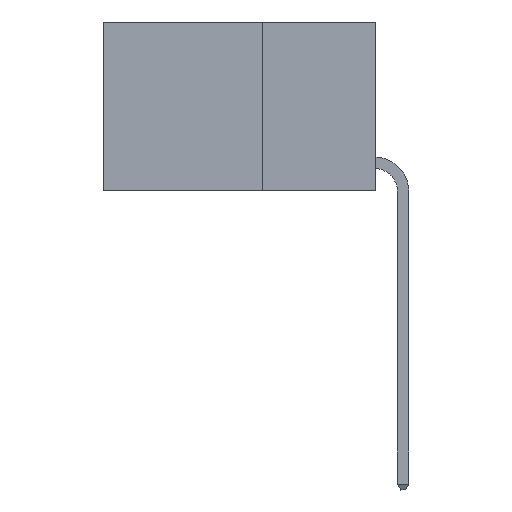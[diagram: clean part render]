
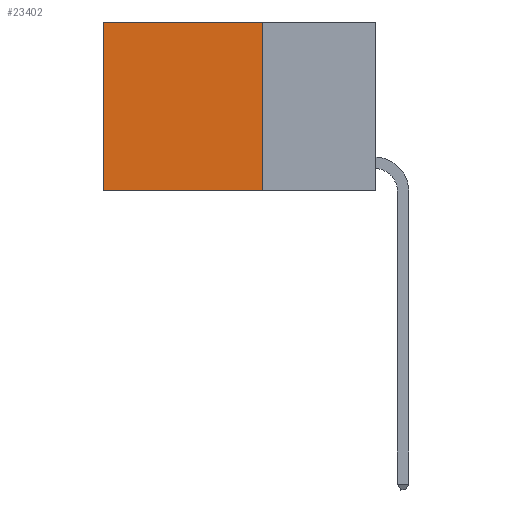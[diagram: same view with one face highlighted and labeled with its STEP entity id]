
A CAD part, left-side view. The second image highlights one B-rep face of the part: STEP entity #23402.
In plain terms, the highlighted planar face has unit normal (-1, 0, 0).
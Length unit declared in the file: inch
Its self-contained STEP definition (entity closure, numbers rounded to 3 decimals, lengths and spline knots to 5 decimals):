
#602 = VECTOR ( 'NONE', #968, 39.37008 ) ;
#740 = CARTESIAN_POINT ( 'NONE',  ( 0.2625, 0.25, -0.37 ) ) ;
#968 = DIRECTION ( 'NONE',  ( 0., 1., 0. ) ) ;
#1025 = LINE ( 'NONE', #740, #27747 ) ;
#2262 = VERTEX_POINT ( 'NONE', #26329 ) ;
#2319 = DIRECTION ( 'NONE',  ( 1., 0., 0. ) ) ;
#2471 = CARTESIAN_POINT ( 'NONE',  ( 0.2625, 0.25, 0. ) ) ;
#3002 = ORIENTED_EDGE ( 'NONE', *, *, #13881, .F. ) ;
#3449 = VECTOR ( 'NONE', #24033, 39.37008 ) ;
#4096 = DIRECTION ( 'NONE',  ( 0., 0., -1. ) ) ;
#4348 = VERTEX_POINT ( 'NONE', #27523 ) ;
#4671 = EDGE_CURVE ( 'NONE', #10564, #2262, #7928, .T. ) ;
#5039 = FACE_OUTER_BOUND ( 'NONE', #18988, .T. ) ;
#5051 = ORIENTED_EDGE ( 'NONE', *, *, #4671, .T. ) ;
#7715 = EDGE_CURVE ( 'NONE', #15222, #10564, #13028, .T. ) ;
#7928 = LINE ( 'NONE', #14986, #3449 ) ;
#8964 = CARTESIAN_POINT ( 'NONE',  ( 0.2625, 0.25, 0. ) ) ;
#10340 = CARTESIAN_POINT ( 'NONE',  ( 0.2625, 0.6, 0. ) ) ;
#10564 = VERTEX_POINT ( 'NONE', #10340 ) ;
#11210 = PLANE ( 'NONE',  #16052 ) ;
#11504 = DIRECTION ( 'NONE',  ( 0., 0., -1. ) ) ;
#13028 = LINE ( 'NONE', #28563, #602 ) ;
#13881 = EDGE_CURVE ( 'NONE', #4348, #2262, #1025, .T. ) ;
#14986 = CARTESIAN_POINT ( 'NONE',  ( 0.2625, 0.6, 0. ) ) ;
#15222 = VERTEX_POINT ( 'NONE', #2471 ) ;
#15369 = EDGE_CURVE ( 'NONE', #15222, #4348, #20830, .T. ) ;
#16052 = AXIS2_PLACEMENT_3D ( 'NONE', #8964, #2319, #11504 ) ;
#18569 = CARTESIAN_POINT ( 'NONE',  ( 0.2625, 0.25, 0. ) ) ;
#18988 = EDGE_LOOP ( 'NONE', ( #5051, #3002, #27911, #24327 ) ) ;
#20830 = LINE ( 'NONE', #18569, #22037 ) ;
#21589 = DIRECTION ( 'NONE',  ( 0., 1., 0. ) ) ;
#22037 = VECTOR ( 'NONE', #4096, 39.37008 ) ;
#23402 = ADVANCED_FACE ( 'NONE', ( #5039 ), #11210, .F. ) ;
#24033 = DIRECTION ( 'NONE',  ( 0., 0., -1. ) ) ;
#24327 = ORIENTED_EDGE ( 'NONE', *, *, #7715, .T. ) ;
#26329 = CARTESIAN_POINT ( 'NONE',  ( 0.2625, 0.6, -0.37 ) ) ;
#27523 = CARTESIAN_POINT ( 'NONE',  ( 0.2625, 0.25, -0.37 ) ) ;
#27747 = VECTOR ( 'NONE', #21589, 39.37008 ) ;
#27911 = ORIENTED_EDGE ( 'NONE', *, *, #15369, .F. ) ;
#28563 = CARTESIAN_POINT ( 'NONE',  ( 0.2625, 0.25, 0. ) ) ;
